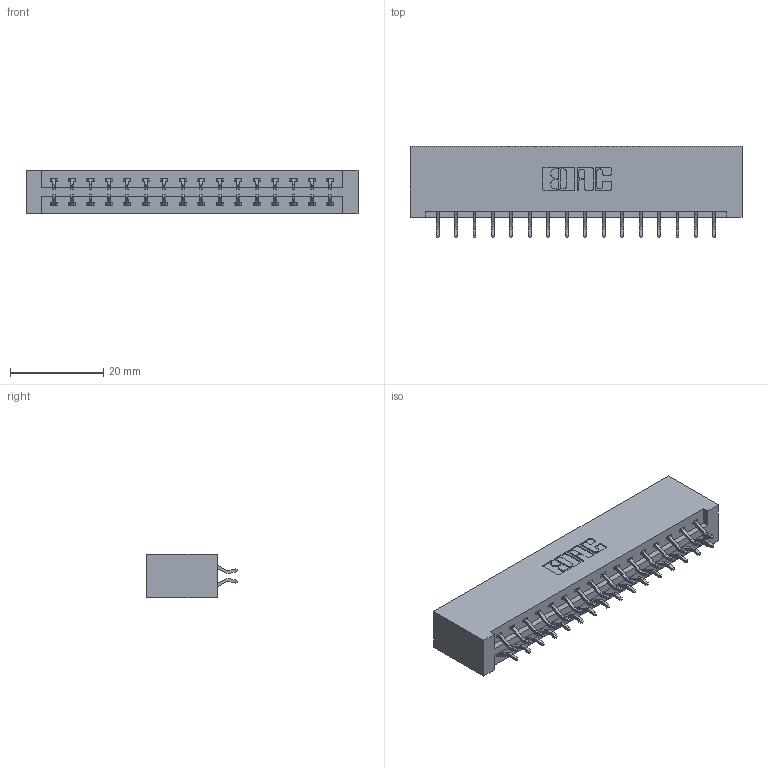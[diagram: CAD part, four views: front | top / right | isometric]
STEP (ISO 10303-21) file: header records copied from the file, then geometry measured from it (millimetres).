
FILE_DESCRIPTION (( 'STEP AP203' ), '1' );
FILE_NAME ('387-032-556-201.STEP', '2018-09-18T08:01:49', ( '' ), ( '' ), 'SwSTEP 2.0', 'SolidWorks 2016', '' );
FILE_SCHEMA (( 'CONFIG_CONTROL_DESIGN' ));
Length unit declared in the file: inch
Products named in the file (3): 337 Part_No Mounting Lugs; 345-292-001_556 Tail; 387-032-556-201
Assembly tree (33 placements, depth 2):
  387-032-556-201
    337 Part_No Mounting Lugs
    345-292-001_556 Tail  x32
Bounding box: 71.27 x 19.57 x 9.4 mm (x, y, z)
Volume: 7924.6 mm3; surface area: 8728.6 mm2
Topology: 33 solids, 33 shells, 2026 faces, 6015 edges, 3966 vertices
Faces by surface type: plane 1410, cylinder 616
Entity records: 15711 total; most frequent: CARTESIAN_POINT 2682, ORIENTED_EDGE 2606, DIRECTION 2311, EDGE_CURVE 1303, VECTOR 1175, LINE 1175, VERTEX_POINT 866, AXIS2_PLACEMENT_3D 568
